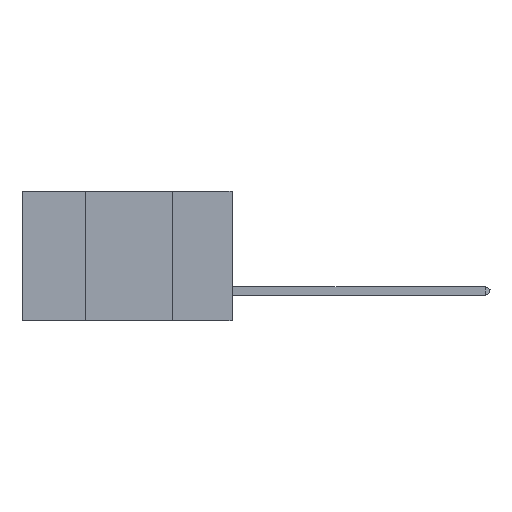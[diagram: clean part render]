
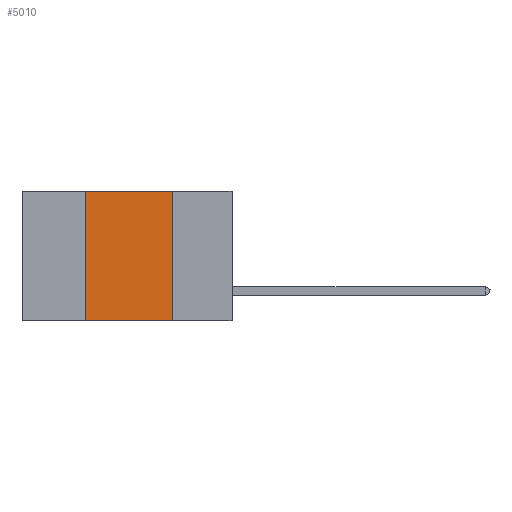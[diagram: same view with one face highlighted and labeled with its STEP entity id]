
A CAD part, left-side view. The second image highlights one B-rep face of the part: STEP entity #5010.
In plain terms, the highlighted planar face has unit normal (-1, 0, 0).
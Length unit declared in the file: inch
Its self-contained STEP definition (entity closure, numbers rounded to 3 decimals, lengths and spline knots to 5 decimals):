
#754 = ORIENTED_EDGE ( 'NONE', *, *, #14304, .T. ) ;
#790 = DIRECTION ( 'NONE',  ( 0., -1., 0. ) ) ;
#1242 = EDGE_LOOP ( 'NONE', ( #2339, #10860, #14752, #754 ) ) ;
#1454 = LINE ( 'NONE', #11477, #7589 ) ;
#1758 = VECTOR ( 'NONE', #3872, 39.37008 ) ;
#1767 = CARTESIAN_POINT ( 'NONE',  ( 0., 0.17, 0. ) ) ;
#2339 = ORIENTED_EDGE ( 'NONE', *, *, #6696, .F. ) ;
#3119 = CARTESIAN_POINT ( 'NONE',  ( 0., 0.17, -0.37 ) ) ;
#3347 = EDGE_CURVE ( 'NONE', #9557, #12087, #6456, .T. ) ;
#3410 = DIRECTION ( 'NONE',  ( 0., 0., -1. ) ) ;
#3872 = DIRECTION ( 'NONE',  ( 0., -1., 0. ) ) ;
#4111 = CARTESIAN_POINT ( 'NONE',  ( 0., 0.42, 0. ) ) ;
#4208 = PLANE ( 'NONE',  #4537 ) ;
#4537 = AXIS2_PLACEMENT_3D ( 'NONE', #4580, #5919, #16534 ) ;
#4564 = VERTEX_POINT ( 'NONE', #3119 ) ;
#4580 = CARTESIAN_POINT ( 'NONE',  ( 0., 0.6, 0. ) ) ;
#4590 = VECTOR ( 'NONE', #16197, 39.37008 ) ;
#5010 = ADVANCED_FACE ( 'NONE', ( #9860 ), #4208, .F. ) ;
#5322 = LINE ( 'NONE', #11926, #1758 ) ;
#5919 = DIRECTION ( 'NONE',  ( 1., 0., 0. ) ) ;
#6456 = LINE ( 'NONE', #4111, #4590 ) ;
#6696 = EDGE_CURVE ( 'NONE', #14112, #4564, #6812, .T. ) ;
#6812 = LINE ( 'NONE', #16837, #11043 ) ;
#7589 = VECTOR ( 'NONE', #790, 39.37008 ) ;
#9557 = VERTEX_POINT ( 'NONE', #11694 ) ;
#9860 = FACE_OUTER_BOUND ( 'NONE', #1242, .T. ) ;
#10860 = ORIENTED_EDGE ( 'NONE', *, *, #16834, .F. ) ;
#11043 = VECTOR ( 'NONE', #3410, 39.37008 ) ;
#11477 = CARTESIAN_POINT ( 'NONE',  ( 0., 0.6, 0. ) ) ;
#11694 = CARTESIAN_POINT ( 'NONE',  ( 0., 0.42, -0.37 ) ) ;
#11926 = CARTESIAN_POINT ( 'NONE',  ( 0., 0.6, -0.37 ) ) ;
#12087 = VERTEX_POINT ( 'NONE', #12895 ) ;
#12895 = CARTESIAN_POINT ( 'NONE',  ( 0., 0.42, 0. ) ) ;
#14112 = VERTEX_POINT ( 'NONE', #1767 ) ;
#14304 = EDGE_CURVE ( 'NONE', #9557, #4564, #5322, .T. ) ;
#14752 = ORIENTED_EDGE ( 'NONE', *, *, #3347, .F. ) ;
#16197 = DIRECTION ( 'NONE',  ( 0., 0., 1. ) ) ;
#16534 = DIRECTION ( 'NONE',  ( 0., 0., -1. ) ) ;
#16834 = EDGE_CURVE ( 'NONE', #12087, #14112, #1454, .T. ) ;
#16837 = CARTESIAN_POINT ( 'NONE',  ( 0., 0.17, 0. ) ) ;
